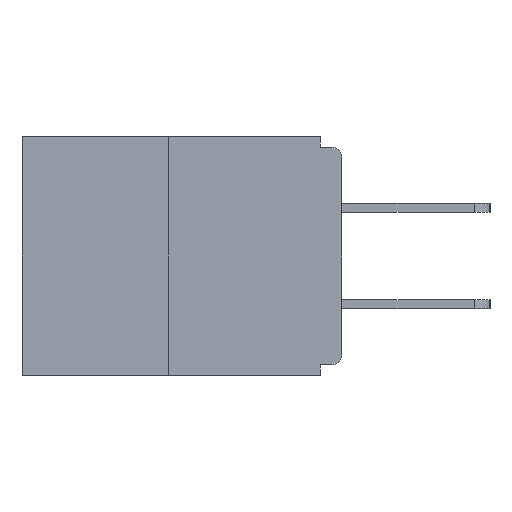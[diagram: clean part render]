
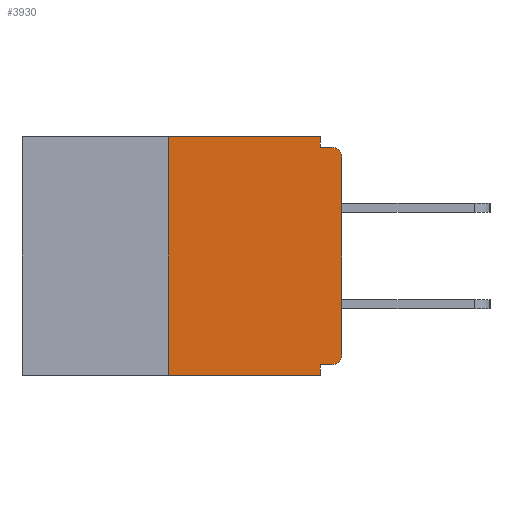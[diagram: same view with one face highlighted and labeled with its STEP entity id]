
A CAD part, left-side view. The second image highlights one B-rep face of the part: STEP entity #3930.
In plain terms, the highlighted planar face has unit normal (-1, 0, 0).
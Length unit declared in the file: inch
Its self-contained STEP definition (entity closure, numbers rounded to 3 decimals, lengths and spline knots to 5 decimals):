
#65 = CARTESIAN_POINT ( 'NONE',  ( 0., 0., -0.03 ) ) ;
#656 = DIRECTION ( 'NONE',  ( 0., -1., 0. ) ) ;
#685 = DIRECTION ( 'NONE',  ( 0., 0., -1. ) ) ;
#842 = EDGE_CURVE ( 'NONE', #21015, #18595, #12471, .T. ) ;
#1385 = LINE ( 'NONE', #19018, #11443 ) ;
#1776 = LINE ( 'NONE', #7327, #19559 ) ;
#2086 = EDGE_CURVE ( 'NONE', #19088, #17455, #10859, .T. ) ;
#2402 = CARTESIAN_POINT ( 'NONE',  ( 0., 0.25, 0. ) ) ;
#2738 = VECTOR ( 'NONE', #656, 39.37008 ) ;
#2755 = VERTEX_POINT ( 'NONE', #4370 ) ;
#2967 = EDGE_CURVE ( 'NONE', #16675, #20457, #13681, .T. ) ;
#3131 = CIRCLE ( 'NONE', #6323, 0.015 ) ;
#3283 = EDGE_CURVE ( 'NONE', #13524, #19757, #1776, .T. ) ;
#3605 = EDGE_CURVE ( 'NONE', #20457, #18595, #8160, .T. ) ;
#3854 = VECTOR ( 'NONE', #685, 39.37008 ) ;
#3930 = ADVANCED_FACE ( 'NONE', ( #10221 ), #10729, .F. ) ;
#4001 = DIRECTION ( 'NONE',  ( 0., 0., 1. ) ) ;
#4280 = DIRECTION ( 'NONE',  ( 0., 0., -1. ) ) ;
#4370 = CARTESIAN_POINT ( 'NONE',  ( 0., 0.015, -0.015 ) ) ;
#5219 = DIRECTION ( 'NONE',  ( 0., -1., 0. ) ) ;
#5446 = ORIENTED_EDGE ( 'NONE', *, *, #14276, .F. ) ;
#5505 = AXIS2_PLACEMENT_3D ( 'NONE', #18992, #9115, #4280 ) ;
#5875 = CARTESIAN_POINT ( 'NONE',  ( 0., 0., -0.015 ) ) ;
#6323 = AXIS2_PLACEMENT_3D ( 'NONE', #16888, #18400, #7016 ) ;
#6706 = CARTESIAN_POINT ( 'NONE',  ( 0., 0.015, -0.313 ) ) ;
#6900 = AXIS2_PLACEMENT_3D ( 'NONE', #6706, #18261, #8369 ) ;
#7016 = DIRECTION ( 'NONE',  ( 0., 0., -1. ) ) ;
#7067 = CARTESIAN_POINT ( 'NONE',  ( 0., 0., -0.313 ) ) ;
#7327 = CARTESIAN_POINT ( 'NONE',  ( 0., 0., 0. ) ) ;
#7362 = DIRECTION ( 'NONE',  ( 0., 1., 0. ) ) ;
#7659 = VECTOR ( 'NONE', #14849, 39.37008 ) ;
#8160 = LINE ( 'NONE', #14632, #7659 ) ;
#8369 = DIRECTION ( 'NONE',  ( 0., 0., -1. ) ) ;
#8385 = EDGE_CURVE ( 'NONE', #16675, #13524, #14114, .T. ) ;
#8819 = CARTESIAN_POINT ( 'NONE',  ( 0., 0.031, -0.328 ) ) ;
#8855 = CARTESIAN_POINT ( 'NONE',  ( 0., 0., -0.328 ) ) ;
#9115 = DIRECTION ( 'NONE',  ( 1., 0., 0. ) ) ;
#9122 = ORIENTED_EDGE ( 'NONE', *, *, #3283, .T. ) ;
#9230 = VECTOR ( 'NONE', #14876, 39.37008 ) ;
#9403 = ORIENTED_EDGE ( 'NONE', *, *, #3605, .F. ) ;
#9843 = VECTOR ( 'NONE', #5219, 39.37008 ) ;
#9850 = CARTESIAN_POINT ( 'NONE',  ( 0., 0.031, -0.015 ) ) ;
#10024 = CARTESIAN_POINT ( 'NONE',  ( 0., 0.015, -0.328 ) ) ;
#10221 = FACE_OUTER_BOUND ( 'NONE', #18785, .T. ) ;
#10729 = PLANE ( 'NONE',  #5505 ) ;
#10782 = ORIENTED_EDGE ( 'NONE', *, *, #16403, .F. ) ;
#10859 = LINE ( 'NONE', #20289, #3854 ) ;
#10959 = ORIENTED_EDGE ( 'NONE', *, *, #2086, .F. ) ;
#11443 = VECTOR ( 'NONE', #19164, 39.37008 ) ;
#11994 = CARTESIAN_POINT ( 'NONE',  ( 0., 0.46, -0.343 ) ) ;
#12471 = LINE ( 'NONE', #11994, #9843 ) ;
#12548 = EDGE_CURVE ( 'NONE', #17455, #2755, #15114, .T. ) ;
#13151 = ORIENTED_EDGE ( 'NONE', *, *, #17578, .T. ) ;
#13406 = VECTOR ( 'NONE', #7362, 39.37008 ) ;
#13524 = VERTEX_POINT ( 'NONE', #7067 ) ;
#13681 = LINE ( 'NONE', #8855, #13406 ) ;
#14059 = ORIENTED_EDGE ( 'NONE', *, *, #842, .T. ) ;
#14114 = CIRCLE ( 'NONE', #6900, 0.015 ) ;
#14276 = EDGE_CURVE ( 'NONE', #21015, #17198, #1385, .T. ) ;
#14632 = CARTESIAN_POINT ( 'NONE',  ( 0., 0.031, -0.343 ) ) ;
#14849 = DIRECTION ( 'NONE',  ( 0., 0., -1. ) ) ;
#14876 = DIRECTION ( 'NONE',  ( 0., -1., 0. ) ) ;
#15108 = CARTESIAN_POINT ( 'NONE',  ( 0., 0.031, -0.343 ) ) ;
#15114 = LINE ( 'NONE', #5875, #2738 ) ;
#16375 = ORIENTED_EDGE ( 'NONE', *, *, #2967, .F. ) ;
#16403 = EDGE_CURVE ( 'NONE', #17198, #19088, #19823, .T. ) ;
#16431 = CARTESIAN_POINT ( 'NONE',  ( 0., 0.46, 0. ) ) ;
#16675 = VERTEX_POINT ( 'NONE', #10024 ) ;
#16888 = CARTESIAN_POINT ( 'NONE',  ( 0., 0.015, -0.03 ) ) ;
#17198 = VERTEX_POINT ( 'NONE', #2402 ) ;
#17455 = VERTEX_POINT ( 'NONE', #9850 ) ;
#17578 = EDGE_CURVE ( 'NONE', #19757, #2755, #3131, .T. ) ;
#18261 = DIRECTION ( 'NONE',  ( -1., 0., 0. ) ) ;
#18400 = DIRECTION ( 'NONE',  ( -1., 0., 0. ) ) ;
#18595 = VERTEX_POINT ( 'NONE', #15108 ) ;
#18704 = CARTESIAN_POINT ( 'NONE',  ( 0., 0.25, -0.343 ) ) ;
#18785 = EDGE_LOOP ( 'NONE', ( #10782, #5446, #14059, #9403, #16375, #21234, #9122, #13151, #19574, #10959 ) ) ;
#18992 = CARTESIAN_POINT ( 'NONE',  ( 0., 0.46, 0. ) ) ;
#18997 = CARTESIAN_POINT ( 'NONE',  ( 0., 0.031, 0. ) ) ;
#19018 = CARTESIAN_POINT ( 'NONE',  ( 0., 0.25, 0. ) ) ;
#19088 = VERTEX_POINT ( 'NONE', #18997 ) ;
#19164 = DIRECTION ( 'NONE',  ( 0., 0., 1. ) ) ;
#19559 = VECTOR ( 'NONE', #4001, 39.37008 ) ;
#19574 = ORIENTED_EDGE ( 'NONE', *, *, #12548, .F. ) ;
#19757 = VERTEX_POINT ( 'NONE', #65 ) ;
#19823 = LINE ( 'NONE', #16431, #9230 ) ;
#20289 = CARTESIAN_POINT ( 'NONE',  ( 0., 0.031, 0. ) ) ;
#20457 = VERTEX_POINT ( 'NONE', #8819 ) ;
#21015 = VERTEX_POINT ( 'NONE', #18704 ) ;
#21234 = ORIENTED_EDGE ( 'NONE', *, *, #8385, .T. ) ;
